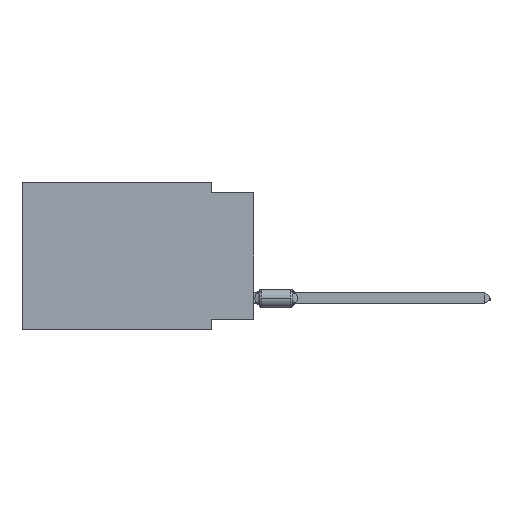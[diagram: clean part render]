
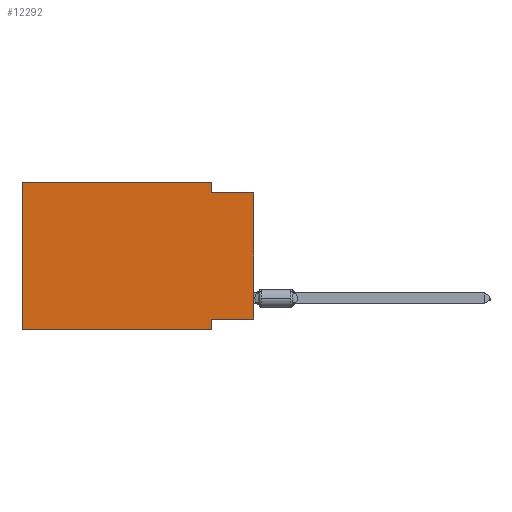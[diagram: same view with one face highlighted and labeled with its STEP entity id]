
A CAD part, left-side view. The second image highlights one B-rep face of the part: STEP entity #12292.
In plain terms, the highlighted planar face has unit normal (-1, 0, 0).
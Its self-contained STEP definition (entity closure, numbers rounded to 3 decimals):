
#1233 = CARTESIAN_POINT ( 'NONE',  ( 0., 13.97, -8.89 ) ) ;
#2636 = EDGE_LOOP ( 'NONE', ( #30423, #41940, #14602, #30143, #12975, #24975, #6287, #41435 ) ) ;
#2651 = FACE_OUTER_BOUND ( 'NONE', #2636, .T. ) ;
#4090 = LINE ( 'NONE', #11243, #44333 ) ;
#5620 = VERTEX_POINT ( 'NONE', #15168 ) ;
#5685 = CARTESIAN_POINT ( 'NONE',  ( 0., 2.54, -0.635 ) ) ;
#6287 = ORIENTED_EDGE ( 'NONE', *, *, #26965, .F. ) ;
#7039 = EDGE_CURVE ( 'NONE', #21169, #34221, #26418, .T. ) ;
#7742 = CARTESIAN_POINT ( 'NONE',  ( 0., 0., -0.635 ) ) ;
#8650 = LINE ( 'NONE', #37006, #23340 ) ;
#10325 = EDGE_CURVE ( 'NONE', #28667, #17136, #13600, .T. ) ;
#10566 = DIRECTION ( 'NONE',  ( 0., 0., 1. ) ) ;
#11243 = CARTESIAN_POINT ( 'NONE',  ( 0., 13.97, 0. ) ) ;
#11403 = VERTEX_POINT ( 'NONE', #25351 ) ;
#11796 = VERTEX_POINT ( 'NONE', #45271 ) ;
#12033 = CARTESIAN_POINT ( 'NONE',  ( 0., 0., -8.255 ) ) ;
#12120 = DIRECTION ( 'NONE',  ( 0., 1., 0. ) ) ;
#12292 = ADVANCED_FACE ( 'NONE', ( #2651 ), #12857, .F. ) ;
#12857 = PLANE ( 'NONE',  #16591 ) ;
#12975 = ORIENTED_EDGE ( 'NONE', *, *, #27273, .F. ) ;
#13600 = LINE ( 'NONE', #27548, #23265 ) ;
#14602 = ORIENTED_EDGE ( 'NONE', *, *, #10325, .F. ) ;
#15168 = CARTESIAN_POINT ( 'NONE',  ( 0., 2.54, -8.255 ) ) ;
#16591 = AXIS2_PLACEMENT_3D ( 'NONE', #23549, #40977, #41206 ) ;
#17136 = VERTEX_POINT ( 'NONE', #5685 ) ;
#17342 = EDGE_CURVE ( 'NONE', #17499, #11796, #40031, .T. ) ;
#17499 = VERTEX_POINT ( 'NONE', #1233 ) ;
#18617 = DIRECTION ( 'NONE',  ( 0., -1., 0. ) ) ;
#19163 = VECTOR ( 'NONE', #12120, 1000. ) ;
#19304 = DIRECTION ( 'NONE',  ( 0., -1., 0. ) ) ;
#21169 = VERTEX_POINT ( 'NONE', #12033 ) ;
#22115 = LINE ( 'NONE', #7742, #27001 ) ;
#22871 = VECTOR ( 'NONE', #18617, 1000. ) ;
#22912 = DIRECTION ( 'NONE',  ( 0., 0., 1. ) ) ;
#23265 = VECTOR ( 'NONE', #41263, 1000. ) ;
#23340 = VECTOR ( 'NONE', #19304, 1000. ) ;
#23549 = CARTESIAN_POINT ( 'NONE',  ( 0., 13.97, 0. ) ) ;
#24975 = ORIENTED_EDGE ( 'NONE', *, *, #17342, .T. ) ;
#25174 = CARTESIAN_POINT ( 'NONE',  ( 0., 13.97, -8.89 ) ) ;
#25351 = CARTESIAN_POINT ( 'NONE',  ( 0., 13.97, 0. ) ) ;
#26418 = LINE ( 'NONE', #40584, #39785 ) ;
#26506 = VECTOR ( 'NONE', #29668, 1000. ) ;
#26619 = LINE ( 'NONE', #40568, #26506 ) ;
#26965 = EDGE_CURVE ( 'NONE', #5620, #11796, #26619, .T. ) ;
#27001 = VECTOR ( 'NONE', #32137, 1000. ) ;
#27221 = CARTESIAN_POINT ( 'NONE',  ( 0., 0., -8.255 ) ) ;
#27273 = EDGE_CURVE ( 'NONE', #17499, #11403, #4090, .T. ) ;
#27548 = CARTESIAN_POINT ( 'NONE',  ( 0., 2.54, 0. ) ) ;
#28667 = VERTEX_POINT ( 'NONE', #45299 ) ;
#29668 = DIRECTION ( 'NONE',  ( 0., 0., -1. ) ) ;
#30143 = ORIENTED_EDGE ( 'NONE', *, *, #31159, .F. ) ;
#30423 = ORIENTED_EDGE ( 'NONE', *, *, #7039, .T. ) ;
#31159 = EDGE_CURVE ( 'NONE', #11403, #28667, #8650, .T. ) ;
#32137 = DIRECTION ( 'NONE',  ( 0., -1., 0. ) ) ;
#34221 = VERTEX_POINT ( 'NONE', #43568 ) ;
#37006 = CARTESIAN_POINT ( 'NONE',  ( 0., 13.97, 0. ) ) ;
#37694 = LINE ( 'NONE', #27221, #19163 ) ;
#39337 = EDGE_CURVE ( 'NONE', #17136, #34221, #22115, .T. ) ;
#39785 = VECTOR ( 'NONE', #22912, 1000. ) ;
#40031 = LINE ( 'NONE', #25174, #22871 ) ;
#40568 = CARTESIAN_POINT ( 'NONE',  ( 0., 2.54, -8.89 ) ) ;
#40584 = CARTESIAN_POINT ( 'NONE',  ( 0., 0., 0. ) ) ;
#40662 = EDGE_CURVE ( 'NONE', #21169, #5620, #37694, .T. ) ;
#40977 = DIRECTION ( 'NONE',  ( 1., 0., 0. ) ) ;
#41206 = DIRECTION ( 'NONE',  ( 0., 0., -1. ) ) ;
#41263 = DIRECTION ( 'NONE',  ( 0., 0., -1. ) ) ;
#41435 = ORIENTED_EDGE ( 'NONE', *, *, #40662, .F. ) ;
#41940 = ORIENTED_EDGE ( 'NONE', *, *, #39337, .F. ) ;
#43568 = CARTESIAN_POINT ( 'NONE',  ( 0., 0., -0.635 ) ) ;
#44333 = VECTOR ( 'NONE', #10566, 1000. ) ;
#45271 = CARTESIAN_POINT ( 'NONE',  ( 0., 2.54, -8.89 ) ) ;
#45299 = CARTESIAN_POINT ( 'NONE',  ( 0., 2.54, 0. ) ) ;
